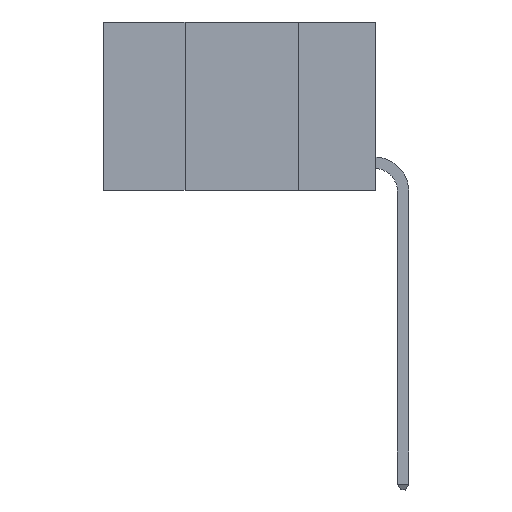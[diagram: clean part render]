
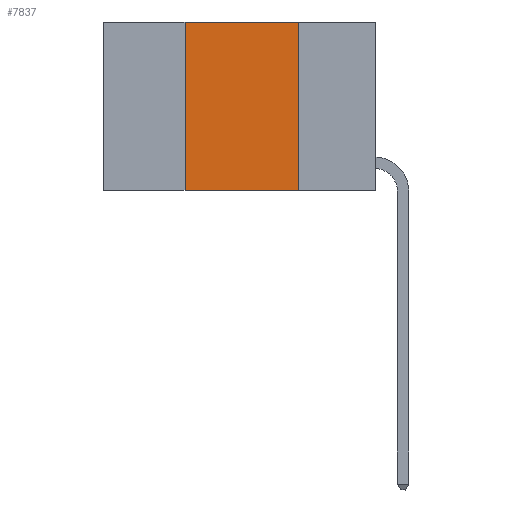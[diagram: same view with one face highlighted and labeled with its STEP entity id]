
A CAD part, left-side view. The second image highlights one B-rep face of the part: STEP entity #7837.
In plain terms, the highlighted planar face has unit normal (-1, 0, 0).
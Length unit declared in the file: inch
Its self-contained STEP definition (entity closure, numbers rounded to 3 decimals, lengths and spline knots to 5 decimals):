
#221 = EDGE_CURVE ( 'NONE', #15656, #5121, #15190, .T. ) ;
#1272 = DIRECTION ( 'NONE',  ( 0., 0., -1. ) ) ;
#1334 = LINE ( 'NONE', #5963, #9661 ) ;
#2090 = CARTESIAN_POINT ( 'NONE',  ( 0., 0.42, 0. ) ) ;
#2536 = EDGE_LOOP ( 'NONE', ( #12665, #16555, #8837, #10124 ) ) ;
#3751 = EDGE_CURVE ( 'NONE', #20176, #5121, #1334, .T. ) ;
#4176 = CARTESIAN_POINT ( 'NONE',  ( 0., 0.6, 0. ) ) ;
#5121 = VERTEX_POINT ( 'NONE', #6193 ) ;
#5140 = LINE ( 'NONE', #8825, #9547 ) ;
#5146 = VECTOR ( 'NONE', #1272, 39.37008 ) ;
#5963 = CARTESIAN_POINT ( 'NONE',  ( 0., 0.6, -0.37 ) ) ;
#6110 = DIRECTION ( 'NONE',  ( 1., 0., 0. ) ) ;
#6159 = EDGE_CURVE ( 'NONE', #16333, #15656, #22749, .T. ) ;
#6193 = CARTESIAN_POINT ( 'NONE',  ( 0., 0.17, -0.37 ) ) ;
#7142 = AXIS2_PLACEMENT_3D ( 'NONE', #4176, #6110, #19231 ) ;
#7602 = EDGE_CURVE ( 'NONE', #20176, #16333, #5140, .T. ) ;
#7626 = CARTESIAN_POINT ( 'NONE',  ( 0., 0.6, 0. ) ) ;
#7837 = ADVANCED_FACE ( 'NONE', ( #9235 ), #15510, .F. ) ;
#8825 = CARTESIAN_POINT ( 'NONE',  ( 0., 0.42, 0. ) ) ;
#8837 = ORIENTED_EDGE ( 'NONE', *, *, #7602, .F. ) ;
#9235 = FACE_OUTER_BOUND ( 'NONE', #2536, .T. ) ;
#9547 = VECTOR ( 'NONE', #21911, 39.37008 ) ;
#9661 = VECTOR ( 'NONE', #19082, 39.37008 ) ;
#10124 = ORIENTED_EDGE ( 'NONE', *, *, #3751, .T. ) ;
#11512 = CARTESIAN_POINT ( 'NONE',  ( 0., 0.17, 0. ) ) ;
#12665 = ORIENTED_EDGE ( 'NONE', *, *, #221, .F. ) ;
#15190 = LINE ( 'NONE', #21704, #5146 ) ;
#15510 = PLANE ( 'NONE',  #7142 ) ;
#15656 = VERTEX_POINT ( 'NONE', #11512 ) ;
#16333 = VERTEX_POINT ( 'NONE', #2090 ) ;
#16555 = ORIENTED_EDGE ( 'NONE', *, *, #6159, .F. ) ;
#17013 = DIRECTION ( 'NONE',  ( 0., -1., 0. ) ) ;
#19082 = DIRECTION ( 'NONE',  ( 0., -1., 0. ) ) ;
#19231 = DIRECTION ( 'NONE',  ( 0., 0., -1. ) ) ;
#19236 = CARTESIAN_POINT ( 'NONE',  ( 0., 0.42, -0.37 ) ) ;
#20176 = VERTEX_POINT ( 'NONE', #19236 ) ;
#21704 = CARTESIAN_POINT ( 'NONE',  ( 0., 0.17, 0. ) ) ;
#21911 = DIRECTION ( 'NONE',  ( 0., 0., 1. ) ) ;
#22158 = VECTOR ( 'NONE', #17013, 39.37008 ) ;
#22749 = LINE ( 'NONE', #7626, #22158 ) ;
